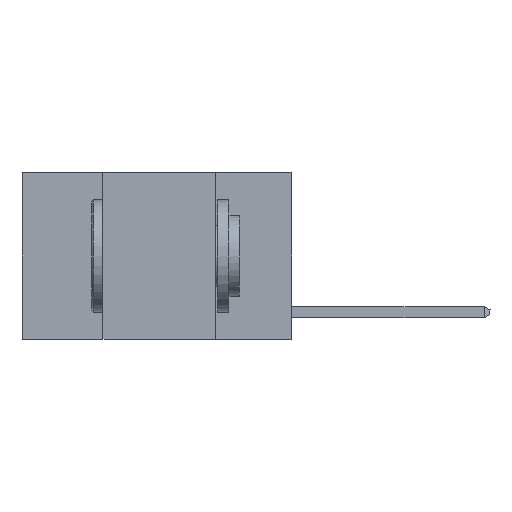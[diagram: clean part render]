
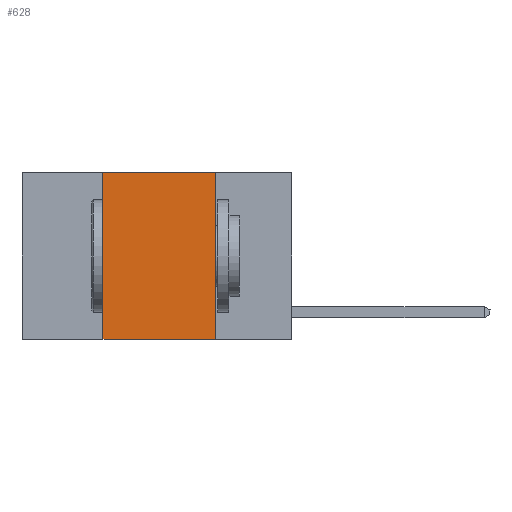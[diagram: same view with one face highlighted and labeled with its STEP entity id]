
A CAD part, left-side view. The second image highlights one B-rep face of the part: STEP entity #628.
In plain terms, the highlighted planar face has unit normal (-1, 0, 0).
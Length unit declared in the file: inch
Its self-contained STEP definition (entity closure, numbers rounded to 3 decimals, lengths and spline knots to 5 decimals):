
#13 = PLANE ( 'NONE',  #11480 ) ;
#130 = CARTESIAN_POINT ( 'NONE',  ( 0., 0.17, -0.37 ) ) ;
#148 = ORIENTED_EDGE ( 'NONE', *, *, #1643, .F. ) ;
#252 = VERTEX_POINT ( 'NONE', #5815 ) ;
#271 = DIRECTION ( 'NONE',  ( 0., -1., 0. ) ) ;
#424 = CARTESIAN_POINT ( 'NONE',  ( 0., 0.6, -0.37 ) ) ;
#613 = DIRECTION ( 'NONE',  ( 0., 0., -1. ) ) ;
#627 = EDGE_CURVE ( 'NONE', #252, #10306, #7321, .T. ) ;
#628 = ADVANCED_FACE ( 'NONE', ( #6754 ), #13, .F. ) ;
#1088 = CARTESIAN_POINT ( 'NONE',  ( 0., 0.42, -0.37 ) ) ;
#1398 = VECTOR ( 'NONE', #10446, 39.37008 ) ;
#1643 = EDGE_CURVE ( 'NONE', #8136, #252, #6430, .T. ) ;
#2248 = EDGE_LOOP ( 'NONE', ( #5494, #11967, #148, #12125 ) ) ;
#2818 = DIRECTION ( 'NONE',  ( 1., 0., 0. ) ) ;
#3574 = CARTESIAN_POINT ( 'NONE',  ( 0., 0.17, 0. ) ) ;
#4652 = DIRECTION ( 'NONE',  ( 0., -1., 0. ) ) ;
#4793 = CARTESIAN_POINT ( 'NONE',  ( 0., 0.42, 0. ) ) ;
#4832 = VECTOR ( 'NONE', #4652, 39.37008 ) ;
#5494 = ORIENTED_EDGE ( 'NONE', *, *, #11202, .F. ) ;
#5815 = CARTESIAN_POINT ( 'NONE',  ( 0., 0.42, 0. ) ) ;
#5830 = LINE ( 'NONE', #6227, #8623 ) ;
#5918 = VERTEX_POINT ( 'NONE', #130 ) ;
#6002 = VECTOR ( 'NONE', #271, 39.37008 ) ;
#6227 = CARTESIAN_POINT ( 'NONE',  ( 0., 0.17, 0. ) ) ;
#6335 = CARTESIAN_POINT ( 'NONE',  ( 0., 0.6, 0. ) ) ;
#6430 = LINE ( 'NONE', #4793, #1398 ) ;
#6754 = FACE_OUTER_BOUND ( 'NONE', #2248, .T. ) ;
#7321 = LINE ( 'NONE', #6335, #4832 ) ;
#8136 = VERTEX_POINT ( 'NONE', #1088 ) ;
#8439 = DIRECTION ( 'NONE',  ( 0., 0., -1. ) ) ;
#8563 = CARTESIAN_POINT ( 'NONE',  ( 0., 0.6, 0. ) ) ;
#8623 = VECTOR ( 'NONE', #613, 39.37008 ) ;
#8882 = EDGE_CURVE ( 'NONE', #8136, #5918, #11048, .T. ) ;
#10306 = VERTEX_POINT ( 'NONE', #3574 ) ;
#10446 = DIRECTION ( 'NONE',  ( 0., 0., 1. ) ) ;
#11048 = LINE ( 'NONE', #424, #6002 ) ;
#11202 = EDGE_CURVE ( 'NONE', #10306, #5918, #5830, .T. ) ;
#11480 = AXIS2_PLACEMENT_3D ( 'NONE', #8563, #2818, #8439 ) ;
#11967 = ORIENTED_EDGE ( 'NONE', *, *, #627, .F. ) ;
#12125 = ORIENTED_EDGE ( 'NONE', *, *, #8882, .T. ) ;
